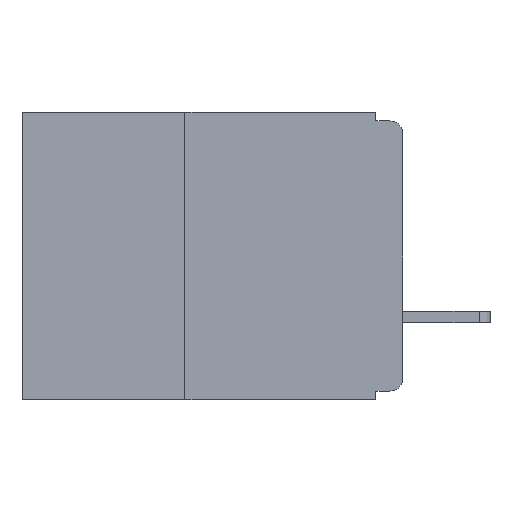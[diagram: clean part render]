
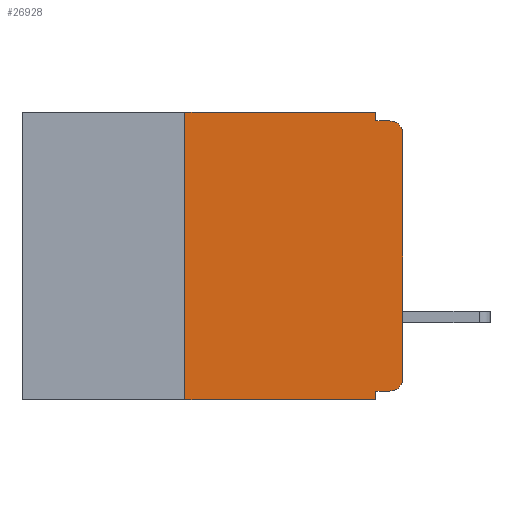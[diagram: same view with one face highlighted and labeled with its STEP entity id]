
A CAD part, left-side view. The second image highlights one B-rep face of the part: STEP entity #26928.
In plain terms, the highlighted planar face has unit normal (-1, 0, 0).
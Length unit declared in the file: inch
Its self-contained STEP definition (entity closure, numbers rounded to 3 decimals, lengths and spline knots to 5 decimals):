
#333 = DIRECTION ( 'NONE',  ( 0., 0., -1. ) ) ;
#613 = VERTEX_POINT ( 'NONE', #18386 ) ;
#1325 = ORIENTED_EDGE ( 'NONE', *, *, #22661, .T. ) ;
#1358 = LINE ( 'NONE', #5920, #6500 ) ;
#1375 = VECTOR ( 'NONE', #19615, 39.37008 ) ;
#1648 = EDGE_CURVE ( 'NONE', #20258, #14473, #20117, .T. ) ;
#1705 = ORIENTED_EDGE ( 'NONE', *, *, #23472, .T. ) ;
#2031 = EDGE_LOOP ( 'NONE', ( #1325, #1705, #5423, #24120, #2516, #10078, #22186, #10358, #16353, #15677 ) ) ;
#2516 = ORIENTED_EDGE ( 'NONE', *, *, #5736, .F. ) ;
#2814 = CIRCLE ( 'NONE', #24723, 0.015 ) ;
#3006 = LINE ( 'NONE', #24036, #19627 ) ;
#3116 = EDGE_CURVE ( 'NONE', #20796, #7383, #10975, .T. ) ;
#3915 = CARTESIAN_POINT ( 'NONE',  ( 0., 0.031, 0. ) ) ;
#5423 = ORIENTED_EDGE ( 'NONE', *, *, #1648, .F. ) ;
#5562 = CARTESIAN_POINT ( 'NONE',  ( 0., 0., -0.305 ) ) ;
#5736 = EDGE_CURVE ( 'NONE', #6199, #15765, #22621, .T. ) ;
#5920 = CARTESIAN_POINT ( 'NONE',  ( 0., 0., -0.32 ) ) ;
#6199 = VERTEX_POINT ( 'NONE', #18987 ) ;
#6482 = CARTESIAN_POINT ( 'NONE',  ( 0., 0.031, 0. ) ) ;
#6500 = VECTOR ( 'NONE', #16736, 39.37008 ) ;
#6683 = VECTOR ( 'NONE', #23509, 39.37008 ) ;
#7383 = VERTEX_POINT ( 'NONE', #19836 ) ;
#7664 = LINE ( 'NONE', #16745, #24171 ) ;
#8029 = CARTESIAN_POINT ( 'NONE',  ( 0., 0.031, -0.33 ) ) ;
#8109 = DIRECTION ( 'NONE',  ( 0., 0., 1. ) ) ;
#8336 = CARTESIAN_POINT ( 'NONE',  ( 0., 0.031, -0.01 ) ) ;
#8601 = CARTESIAN_POINT ( 'NONE',  ( 0., 0., -0.025 ) ) ;
#8986 = LINE ( 'NONE', #3915, #26081 ) ;
#8993 = DIRECTION ( 'NONE',  ( 0., 0., 1. ) ) ;
#9528 = DIRECTION ( 'NONE',  ( 1., 0., 0. ) ) ;
#10078 = ORIENTED_EDGE ( 'NONE', *, *, #17122, .F. ) ;
#10358 = ORIENTED_EDGE ( 'NONE', *, *, #22020, .F. ) ;
#10975 = LINE ( 'NONE', #27288, #1375 ) ;
#11282 = DIRECTION ( 'NONE',  ( -1., 0., 0. ) ) ;
#12167 = AXIS2_PLACEMENT_3D ( 'NONE', #26212, #13447, #333 ) ;
#12190 = CARTESIAN_POINT ( 'NONE',  ( 0., 0.015, -0.01 ) ) ;
#12494 = LINE ( 'NONE', #8029, #6683 ) ;
#13447 = DIRECTION ( 'NONE',  ( -1., 0., 0. ) ) ;
#14473 = VERTEX_POINT ( 'NONE', #12190 ) ;
#15677 = ORIENTED_EDGE ( 'NONE', *, *, #25289, .T. ) ;
#15765 = VERTEX_POINT ( 'NONE', #6482 ) ;
#16353 = ORIENTED_EDGE ( 'NONE', *, *, #19607, .F. ) ;
#16736 = DIRECTION ( 'NONE',  ( 0., 1., 0. ) ) ;
#16745 = CARTESIAN_POINT ( 'NONE',  ( 0., 0., 0. ) ) ;
#17122 = EDGE_CURVE ( 'NONE', #20796, #6199, #3006, .T. ) ;
#17381 = VERTEX_POINT ( 'NONE', #8601 ) ;
#18166 = PLANE ( 'NONE',  #25812 ) ;
#18291 = CARTESIAN_POINT ( 'NONE',  ( 0., 0.031, -0.32 ) ) ;
#18386 = CARTESIAN_POINT ( 'NONE',  ( 0., 0.015, -0.32 ) ) ;
#18987 = CARTESIAN_POINT ( 'NONE',  ( 0., 0.25, 0. ) ) ;
#19093 = DIRECTION ( 'NONE',  ( 0., 0., -1. ) ) ;
#19183 = CARTESIAN_POINT ( 'NONE',  ( 0., 0.437, 0. ) ) ;
#19331 = DIRECTION ( 'NONE',  ( 0., -1., 0. ) ) ;
#19607 = EDGE_CURVE ( 'NONE', #613, #21869, #1358, .T. ) ;
#19615 = DIRECTION ( 'NONE',  ( 0., -1., 0. ) ) ;
#19627 = VECTOR ( 'NONE', #8993, 39.37008 ) ;
#19770 = CIRCLE ( 'NONE', #12167, 0.015 ) ;
#19836 = CARTESIAN_POINT ( 'NONE',  ( 0., 0.031, -0.33 ) ) ;
#20117 = LINE ( 'NONE', #24714, #20801 ) ;
#20258 = VERTEX_POINT ( 'NONE', #8336 ) ;
#20573 = VECTOR ( 'NONE', #19331, 39.37008 ) ;
#20796 = VERTEX_POINT ( 'NONE', #25109 ) ;
#20801 = VECTOR ( 'NONE', #24567, 39.37008 ) ;
#21869 = VERTEX_POINT ( 'NONE', #18291 ) ;
#21945 = VERTEX_POINT ( 'NONE', #5562 ) ;
#22020 = EDGE_CURVE ( 'NONE', #21869, #7383, #12494, .T. ) ;
#22186 = ORIENTED_EDGE ( 'NONE', *, *, #3116, .T. ) ;
#22409 = CARTESIAN_POINT ( 'NONE',  ( 0., 0.437, 0. ) ) ;
#22621 = LINE ( 'NONE', #19183, #20573 ) ;
#22661 = EDGE_CURVE ( 'NONE', #21945, #17381, #7664, .T. ) ;
#23472 = EDGE_CURVE ( 'NONE', #17381, #14473, #19770, .T. ) ;
#23509 = DIRECTION ( 'NONE',  ( 0., 0., -1. ) ) ;
#24036 = CARTESIAN_POINT ( 'NONE',  ( 0., 0.25, -0.33 ) ) ;
#24114 = CARTESIAN_POINT ( 'NONE',  ( 0., 0.015, -0.305 ) ) ;
#24120 = ORIENTED_EDGE ( 'NONE', *, *, #25100, .F. ) ;
#24171 = VECTOR ( 'NONE', #8109, 39.37008 ) ;
#24542 = DIRECTION ( 'NONE',  ( 0., 0., -1. ) ) ;
#24567 = DIRECTION ( 'NONE',  ( 0., -1., 0. ) ) ;
#24714 = CARTESIAN_POINT ( 'NONE',  ( 0., 0., -0.01 ) ) ;
#24723 = AXIS2_PLACEMENT_3D ( 'NONE', #24114, #11282, #26206 ) ;
#25100 = EDGE_CURVE ( 'NONE', #15765, #20258, #8986, .T. ) ;
#25109 = CARTESIAN_POINT ( 'NONE',  ( 0., 0.25, -0.33 ) ) ;
#25289 = EDGE_CURVE ( 'NONE', #613, #21945, #2814, .T. ) ;
#25623 = FACE_OUTER_BOUND ( 'NONE', #2031, .T. ) ;
#25812 = AXIS2_PLACEMENT_3D ( 'NONE', #22409, #9528, #24542 ) ;
#26081 = VECTOR ( 'NONE', #19093, 39.37008 ) ;
#26206 = DIRECTION ( 'NONE',  ( 0., 0., -1. ) ) ;
#26212 = CARTESIAN_POINT ( 'NONE',  ( 0., 0.015, -0.025 ) ) ;
#26928 = ADVANCED_FACE ( 'NONE', ( #25623 ), #18166, .F. ) ;
#27288 = CARTESIAN_POINT ( 'NONE',  ( 0., 0.437, -0.33 ) ) ;
